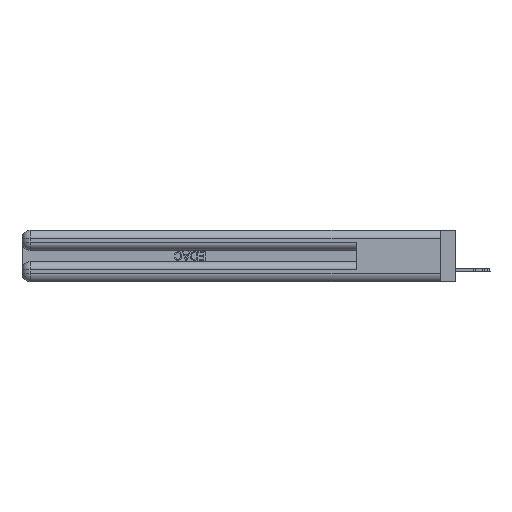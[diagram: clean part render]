
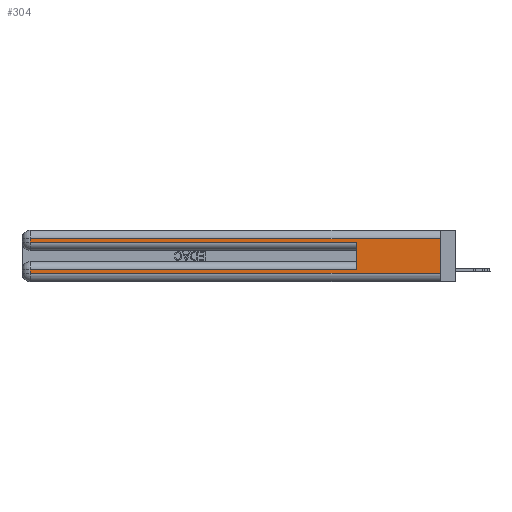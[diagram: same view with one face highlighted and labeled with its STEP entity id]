
A CAD part, left-side view. The second image highlights one B-rep face of the part: STEP entity #304.
In plain terms, the highlighted planar face has unit normal (-1, 0, 0).
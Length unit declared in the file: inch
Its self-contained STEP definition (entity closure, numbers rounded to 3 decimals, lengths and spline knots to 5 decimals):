
#304 = ADVANCED_FACE ( 'NONE', ( #33636 ), #2434, .F. ) ;
#1713 = VECTOR ( 'NONE', #8139, 39.37008 ) ;
#2018 = VECTOR ( 'NONE', #40925, 39.37008 ) ;
#2434 = PLANE ( 'NONE',  #4210 ) ;
#3314 = ORIENTED_EDGE ( 'NONE', *, *, #34749, .T. ) ;
#4210 = AXIS2_PLACEMENT_3D ( 'NONE', #18033, #29316, #6595 ) ;
#4556 = DIRECTION ( 'NONE',  ( 0., 1., 0. ) ) ;
#5044 = CARTESIAN_POINT ( 'NONE',  ( 0., 2.94, 0.06 ) ) ;
#5238 = CARTESIAN_POINT ( 'NONE',  ( 0., 2.94, 0.085 ) ) ;
#5467 = LINE ( 'NONE', #35122, #38192 ) ;
#5833 = LINE ( 'NONE', #25808, #8786 ) ;
#6420 = EDGE_LOOP ( 'NONE', ( #27694, #21412, #45062, #40361, #10948, #48632, #27397, #3314 ) ) ;
#6595 = DIRECTION ( 'NONE',  ( 0., 0., -1. ) ) ;
#6692 = CARTESIAN_POINT ( 'NONE',  ( 0., 0.6, 0.285 ) ) ;
#6696 = CARTESIAN_POINT ( 'NONE',  ( 0., 0.6, 0.085 ) ) ;
#8139 = DIRECTION ( 'NONE',  ( 0., -1., 0. ) ) ;
#8232 = EDGE_CURVE ( 'NONE', #21468, #22468, #13881, .T. ) ;
#8506 = LINE ( 'NONE', #27306, #13920 ) ;
#8786 = VECTOR ( 'NONE', #18344, 39.37008 ) ;
#10308 = EDGE_CURVE ( 'NONE', #48103, #40884, #21497, .T. ) ;
#10948 = ORIENTED_EDGE ( 'NONE', *, *, #20081, .F. ) ;
#11406 = VECTOR ( 'NONE', #33236, 39.37008 ) ;
#13447 = CARTESIAN_POINT ( 'NONE',  ( 0., 2.94, 0.285 ) ) ;
#13692 = VERTEX_POINT ( 'NONE', #6696 ) ;
#13881 = LINE ( 'NONE', #48833, #47787 ) ;
#13920 = VECTOR ( 'NONE', #20191, 39.37008 ) ;
#17857 = CARTESIAN_POINT ( 'NONE',  ( 0., 0., 0.31 ) ) ;
#18033 = CARTESIAN_POINT ( 'NONE',  ( 0., 0., 0.37 ) ) ;
#18344 = DIRECTION ( 'NONE',  ( 0., 0., 1. ) ) ;
#19502 = VERTEX_POINT ( 'NONE', #17857 ) ;
#19786 = LINE ( 'NONE', #37580, #2018 ) ;
#20081 = EDGE_CURVE ( 'NONE', #13692, #48705, #5833, .T. ) ;
#20191 = DIRECTION ( 'NONE',  ( 0., 0., -1. ) ) ;
#21412 = ORIENTED_EDGE ( 'NONE', *, *, #27106, .T. ) ;
#21468 = VERTEX_POINT ( 'NONE', #5238 ) ;
#21497 = LINE ( 'NONE', #43891, #11406 ) ;
#22067 = DIRECTION ( 'NONE',  ( 0., 1., 0. ) ) ;
#22468 = VERTEX_POINT ( 'NONE', #5044 ) ;
#23693 = VECTOR ( 'NONE', #22067, 39.37008 ) ;
#24433 = VERTEX_POINT ( 'NONE', #43178 ) ;
#25808 = CARTESIAN_POINT ( 'NONE',  ( 0., 0.6, 0.145 ) ) ;
#26209 = EDGE_CURVE ( 'NONE', #19502, #24433, #8506, .T. ) ;
#27106 = EDGE_CURVE ( 'NONE', #19502, #48103, #5467, .T. ) ;
#27306 = CARTESIAN_POINT ( 'NONE',  ( 0., 0., 0.37 ) ) ;
#27397 = ORIENTED_EDGE ( 'NONE', *, *, #8232, .T. ) ;
#27694 = ORIENTED_EDGE ( 'NONE', *, *, #26209, .F. ) ;
#29316 = DIRECTION ( 'NONE',  ( 1., 0., 0. ) ) ;
#30864 = EDGE_CURVE ( 'NONE', #13692, #21468, #33915, .T. ) ;
#32874 = CARTESIAN_POINT ( 'NONE',  ( 0., 2.94, 0.31 ) ) ;
#33236 = DIRECTION ( 'NONE',  ( 0., 0., -1. ) ) ;
#33636 = FACE_OUTER_BOUND ( 'NONE', #6420, .T. ) ;
#33915 = LINE ( 'NONE', #45074, #23693 ) ;
#34749 = EDGE_CURVE ( 'NONE', #22468, #24433, #42770, .T. ) ;
#35122 = CARTESIAN_POINT ( 'NONE',  ( 0., 0., 0.31 ) ) ;
#37580 = CARTESIAN_POINT ( 'NONE',  ( 0., 0., 0.285 ) ) ;
#38140 = EDGE_CURVE ( 'NONE', #40884, #48705, #19786, .T. ) ;
#38192 = VECTOR ( 'NONE', #4556, 39.37008 ) ;
#38439 = CARTESIAN_POINT ( 'NONE',  ( 0., 0., 0.06 ) ) ;
#40361 = ORIENTED_EDGE ( 'NONE', *, *, #38140, .T. ) ;
#40884 = VERTEX_POINT ( 'NONE', #13447 ) ;
#40925 = DIRECTION ( 'NONE',  ( 0., -1., 0. ) ) ;
#42770 = LINE ( 'NONE', #38439, #1713 ) ;
#43178 = CARTESIAN_POINT ( 'NONE',  ( 0., 0., 0.06 ) ) ;
#43891 = CARTESIAN_POINT ( 'NONE',  ( 0., 2.94, 0.37 ) ) ;
#45062 = ORIENTED_EDGE ( 'NONE', *, *, #10308, .T. ) ;
#45074 = CARTESIAN_POINT ( 'NONE',  ( 0., 0., 0.085 ) ) ;
#47787 = VECTOR ( 'NONE', #48318, 39.37008 ) ;
#48103 = VERTEX_POINT ( 'NONE', #32874 ) ;
#48318 = DIRECTION ( 'NONE',  ( 0., 0., -1. ) ) ;
#48632 = ORIENTED_EDGE ( 'NONE', *, *, #30864, .T. ) ;
#48705 = VERTEX_POINT ( 'NONE', #6692 ) ;
#48833 = CARTESIAN_POINT ( 'NONE',  ( 0., 2.94, 0.37 ) ) ;
